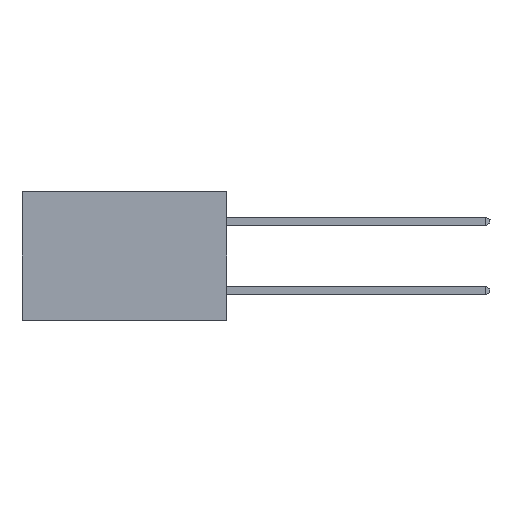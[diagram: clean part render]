
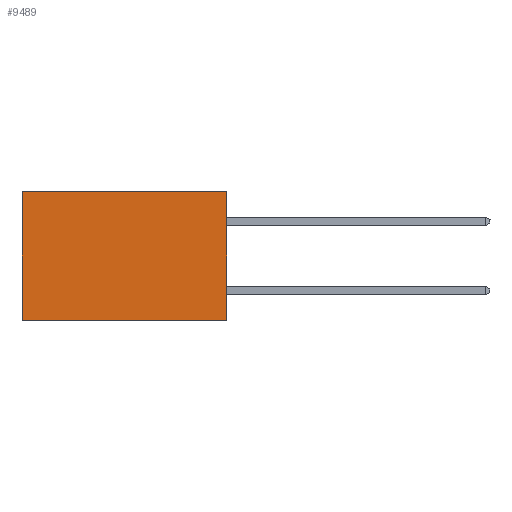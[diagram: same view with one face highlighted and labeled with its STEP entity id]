
A CAD part, left-side view. The second image highlights one B-rep face of the part: STEP entity #9489.
In plain terms, the highlighted planar face has unit normal (-1, 0, 0).
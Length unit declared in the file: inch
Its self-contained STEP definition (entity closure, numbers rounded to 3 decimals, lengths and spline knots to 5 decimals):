
#281 = CARTESIAN_POINT ( 'NONE',  ( 0.277, 0.59, 0. ) ) ;
#1895 = VECTOR ( 'NONE', #15095, 39.37008 ) ;
#2988 = EDGE_CURVE ( 'NONE', #8570, #17087, #12799, .T. ) ;
#3180 = LINE ( 'NONE', #13782, #1895 ) ;
#4072 = ORIENTED_EDGE ( 'NONE', *, *, #4174, .T. ) ;
#4174 = EDGE_CURVE ( 'NONE', #15298, #7226, #6299, .T. ) ;
#4279 = CARTESIAN_POINT ( 'NONE',  ( 0.277, 0.59, -0.37 ) ) ;
#5567 = PLANE ( 'NONE',  #13502 ) ;
#5884 = VECTOR ( 'NONE', #11432, 39.37008 ) ;
#6292 = ORIENTED_EDGE ( 'NONE', *, *, #2988, .F. ) ;
#6299 = LINE ( 'NONE', #11135, #5884 ) ;
#6616 = CARTESIAN_POINT ( 'NONE',  ( 0.277, 0.59, -0.37 ) ) ;
#6725 = DIRECTION ( 'NONE',  ( 0., 0., -1. ) ) ;
#6964 = DIRECTION ( 'NONE',  ( 1., 0., 0. ) ) ;
#7226 = VERTEX_POINT ( 'NONE', #281 ) ;
#7620 = LINE ( 'NONE', #6616, #11216 ) ;
#8311 = EDGE_CURVE ( 'NONE', #7226, #17087, #7620, .T. ) ;
#8570 = VERTEX_POINT ( 'NONE', #15796 ) ;
#8899 = EDGE_CURVE ( 'NONE', #15298, #8570, #3180, .T. ) ;
#9489 = ADVANCED_FACE ( 'NONE', ( #10513 ), #5567, .F. ) ;
#10249 = EDGE_LOOP ( 'NONE', ( #13332, #6292, #13954, #4072 ) ) ;
#10513 = FACE_OUTER_BOUND ( 'NONE', #10249, .T. ) ;
#10963 = CARTESIAN_POINT ( 'NONE',  ( 0.277, 0., -0.37 ) ) ;
#11135 = CARTESIAN_POINT ( 'NONE',  ( 0.277, 0., 0. ) ) ;
#11216 = VECTOR ( 'NONE', #6725, 39.37008 ) ;
#11432 = DIRECTION ( 'NONE',  ( 0., 1., 0. ) ) ;
#12799 = LINE ( 'NONE', #15523, #15867 ) ;
#13332 = ORIENTED_EDGE ( 'NONE', *, *, #8311, .T. ) ;
#13502 = AXIS2_PLACEMENT_3D ( 'NONE', #10963, #6964, #16275 ) ;
#13782 = CARTESIAN_POINT ( 'NONE',  ( 0.277, 0., -0.37 ) ) ;
#13954 = ORIENTED_EDGE ( 'NONE', *, *, #8899, .F. ) ;
#13995 = CARTESIAN_POINT ( 'NONE',  ( 0.277, 0., 0. ) ) ;
#15095 = DIRECTION ( 'NONE',  ( 0., 0., -1. ) ) ;
#15298 = VERTEX_POINT ( 'NONE', #13995 ) ;
#15523 = CARTESIAN_POINT ( 'NONE',  ( 0.277, 0., -0.37 ) ) ;
#15796 = CARTESIAN_POINT ( 'NONE',  ( 0.277, 0., -0.37 ) ) ;
#15867 = VECTOR ( 'NONE', #16128, 39.37008 ) ;
#16128 = DIRECTION ( 'NONE',  ( 0., 1., 0. ) ) ;
#16275 = DIRECTION ( 'NONE',  ( 0., 0., -1. ) ) ;
#17087 = VERTEX_POINT ( 'NONE', #4279 ) ;
